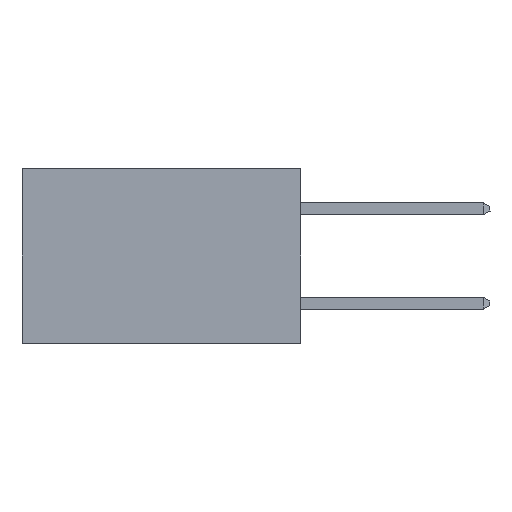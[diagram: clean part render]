
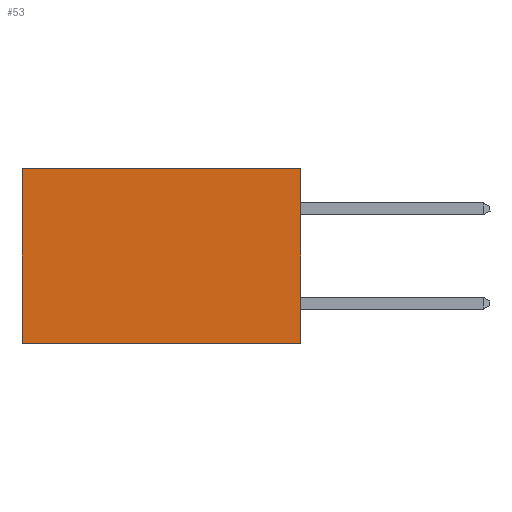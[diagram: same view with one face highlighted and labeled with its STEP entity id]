
A CAD part, left-side view. The second image highlights one B-rep face of the part: STEP entity #53.
In plain terms, the highlighted planar face has unit normal (-1, 0, 0).
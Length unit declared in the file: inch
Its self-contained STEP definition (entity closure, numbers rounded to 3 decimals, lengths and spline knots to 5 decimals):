
#53 = ADVANCED_FACE ( 'NONE', ( #2693 ), #6177, .F. ) ;
#116 = VERTEX_POINT ( 'NONE', #4692 ) ;
#253 = VECTOR ( 'NONE', #569, 39.37008 ) ;
#387 = LINE ( 'NONE', #916, #4888 ) ;
#569 = DIRECTION ( 'NONE',  ( 0., 1., 0. ) ) ;
#635 = CARTESIAN_POINT ( 'NONE',  ( 0.277, 0., 0. ) ) ;
#916 = CARTESIAN_POINT ( 'NONE',  ( 0.277, 0., -0.37 ) ) ;
#961 = DIRECTION ( 'NONE',  ( 0., 1., 0. ) ) ;
#1390 = ORIENTED_EDGE ( 'NONE', *, *, #6773, .T. ) ;
#1634 = VERTEX_POINT ( 'NONE', #5499 ) ;
#1692 = CARTESIAN_POINT ( 'NONE',  ( 0.277, 0., -0.37 ) ) ;
#1909 = LINE ( 'NONE', #635, #253 ) ;
#2131 = VECTOR ( 'NONE', #3991, 39.37008 ) ;
#2178 = CARTESIAN_POINT ( 'NONE',  ( 0.277, 0.59, -0.37 ) ) ;
#2287 = VERTEX_POINT ( 'NONE', #2772 ) ;
#2436 = DIRECTION ( 'NONE',  ( 0., 0., -1. ) ) ;
#2485 = LINE ( 'NONE', #4257, #2131 ) ;
#2693 = FACE_OUTER_BOUND ( 'NONE', #2740, .T. ) ;
#2740 = EDGE_LOOP ( 'NONE', ( #5633, #7147, #7300, #1390 ) ) ;
#2772 = CARTESIAN_POINT ( 'NONE',  ( 0.277, 0., 0. ) ) ;
#3991 = DIRECTION ( 'NONE',  ( 0., 0., -1. ) ) ;
#4257 = CARTESIAN_POINT ( 'NONE',  ( 0.277, 0., -0.37 ) ) ;
#4678 = LINE ( 'NONE', #2178, #7479 ) ;
#4692 = CARTESIAN_POINT ( 'NONE',  ( 0.277, 0.59, 0. ) ) ;
#4745 = DIRECTION ( 'NONE',  ( 1., 0., 0. ) ) ;
#4855 = VERTEX_POINT ( 'NONE', #1692 ) ;
#4888 = VECTOR ( 'NONE', #961, 39.37008 ) ;
#4941 = EDGE_CURVE ( 'NONE', #4855, #1634, #387, .T. ) ;
#5081 = EDGE_CURVE ( 'NONE', #2287, #4855, #2485, .T. ) ;
#5480 = CARTESIAN_POINT ( 'NONE',  ( 0.277, 0., -0.37 ) ) ;
#5499 = CARTESIAN_POINT ( 'NONE',  ( 0.277, 0.59, -0.37 ) ) ;
#5524 = AXIS2_PLACEMENT_3D ( 'NONE', #5480, #4745, #7375 ) ;
#5633 = ORIENTED_EDGE ( 'NONE', *, *, #6582, .T. ) ;
#6177 = PLANE ( 'NONE',  #5524 ) ;
#6582 = EDGE_CURVE ( 'NONE', #116, #1634, #4678, .T. ) ;
#6773 = EDGE_CURVE ( 'NONE', #2287, #116, #1909, .T. ) ;
#7147 = ORIENTED_EDGE ( 'NONE', *, *, #4941, .F. ) ;
#7300 = ORIENTED_EDGE ( 'NONE', *, *, #5081, .F. ) ;
#7375 = DIRECTION ( 'NONE',  ( 0., 0., -1. ) ) ;
#7479 = VECTOR ( 'NONE', #2436, 39.37008 ) ;
